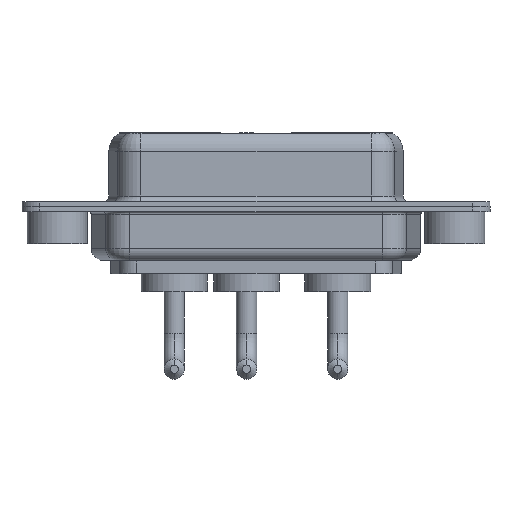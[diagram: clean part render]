
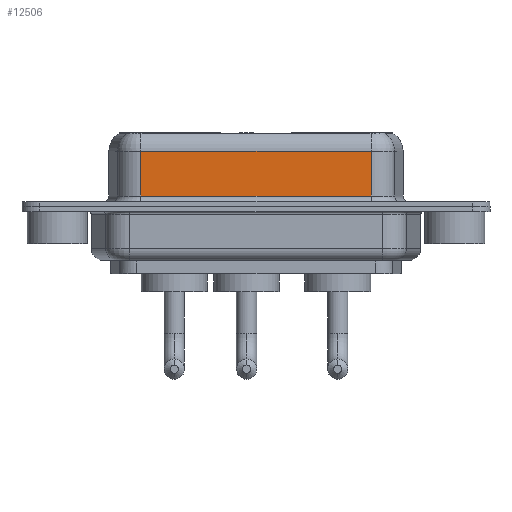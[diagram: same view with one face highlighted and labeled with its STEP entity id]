
A CAD part, front view. The second image highlights one B-rep face of the part: STEP entity #12506.
In plain terms, the highlighted planar face has unit normal (0, -1, 0).
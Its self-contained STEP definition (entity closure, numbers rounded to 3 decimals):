
#962 = DIRECTION ( 'NONE',  ( 0., 1., 0. ) ) ;
#1023 = LINE ( 'NONE', #10673, #2496 ) ;
#1226 = AXIS2_PLACEMENT_3D ( 'NONE', #10282, #962, #9370 ) ;
#1246 = ORIENTED_EDGE ( 'NONE', *, *, #7649, .T. ) ;
#1468 = EDGE_CURVE ( 'NONE', #5575, #11507, #12975, .T. ) ;
#1557 = VERTEX_POINT ( 'NONE', #13449 ) ;
#1962 = VERTEX_POINT ( 'NONE', #4820 ) ;
#2496 = VECTOR ( 'NONE', #12869, 1000. ) ;
#2941 = VECTOR ( 'NONE', #7641, 1000. ) ;
#3101 = ORIENTED_EDGE ( 'NONE', *, *, #3806, .T. ) ;
#3308 = ORIENTED_EDGE ( 'NONE', *, *, #1468, .T. ) ;
#3806 = EDGE_CURVE ( 'NONE', #1962, #5575, #13054, .T. ) ;
#3927 = EDGE_LOOP ( 'NONE', ( #12423, #3101, #3308, #1246 ) ) ;
#4094 = VECTOR ( 'NONE', #13759, 1000. ) ;
#4572 = DIRECTION ( 'NONE',  ( -1., 0., 0. ) ) ;
#4820 = CARTESIAN_POINT ( 'NONE',  ( 26.287, -3.95, 4.65 ) ) ;
#5575 = VERTEX_POINT ( 'NONE', #12260 ) ;
#5743 = CARTESIAN_POINT ( 'NONE',  ( 26.287, -3.95, 4.65 ) ) ;
#6049 = FACE_OUTER_BOUND ( 'NONE', #3927, .T. ) ;
#6444 = VECTOR ( 'NONE', #4572, 1000. ) ;
#7641 = DIRECTION ( 'NONE',  ( 0., 0., -1. ) ) ;
#7649 = EDGE_CURVE ( 'NONE', #11507, #1557, #1023, .T. ) ;
#8445 = CARTESIAN_POINT ( 'NONE',  ( 7.013, -3.95, 0.9 ) ) ;
#8691 = CARTESIAN_POINT ( 'NONE',  ( 7.013, -3.95, 6.4 ) ) ;
#9370 = DIRECTION ( 'NONE',  ( 0., 0., 1. ) ) ;
#10282 = CARTESIAN_POINT ( 'NONE',  ( 26.287, -3.95, 6.4 ) ) ;
#10454 = LINE ( 'NONE', #11805, #4094 ) ;
#10673 = CARTESIAN_POINT ( 'NONE',  ( 26.287, -3.95, 0.9 ) ) ;
#11507 = VERTEX_POINT ( 'NONE', #8445 ) ;
#11805 = CARTESIAN_POINT ( 'NONE',  ( 26.287, -3.95, 6.4 ) ) ;
#11847 = EDGE_CURVE ( 'NONE', #1962, #1557, #10454, .T. ) ;
#12260 = CARTESIAN_POINT ( 'NONE',  ( 7.013, -3.95, 4.65 ) ) ;
#12423 = ORIENTED_EDGE ( 'NONE', *, *, #11847, .F. ) ;
#12506 = ADVANCED_FACE ( 'NONE', ( #6049 ), #13436, .F. ) ;
#12869 = DIRECTION ( 'NONE',  ( 1., 0., 0. ) ) ;
#12975 = LINE ( 'NONE', #8691, #2941 ) ;
#13054 = LINE ( 'NONE', #5743, #6444 ) ;
#13436 = PLANE ( 'NONE',  #1226 ) ;
#13449 = CARTESIAN_POINT ( 'NONE',  ( 26.287, -3.95, 0.9 ) ) ;
#13759 = DIRECTION ( 'NONE',  ( 0., 0., -1. ) ) ;
